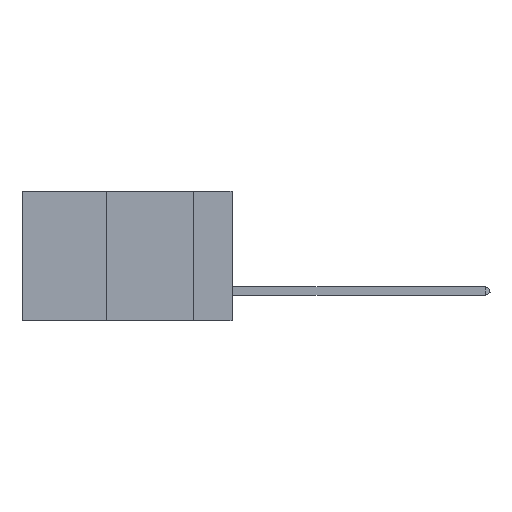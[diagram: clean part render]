
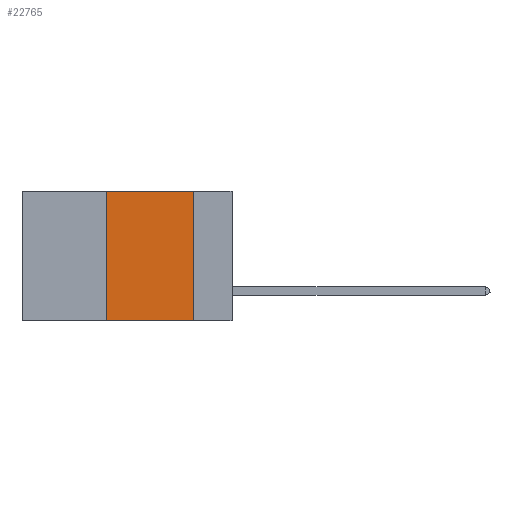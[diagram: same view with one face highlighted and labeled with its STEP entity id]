
A CAD part, left-side view. The second image highlights one B-rep face of the part: STEP entity #22765.
In plain terms, the highlighted planar face has unit normal (-1, 0, 0).
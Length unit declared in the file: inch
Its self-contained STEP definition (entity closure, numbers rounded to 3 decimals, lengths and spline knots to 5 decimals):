
#285 = CARTESIAN_POINT ( 'NONE',  ( 0., 0.36, 0. ) ) ;
#1268 = EDGE_CURVE ( 'NONE', #4175, #27705, #3496, .T. ) ;
#1612 = ORIENTED_EDGE ( 'NONE', *, *, #19260, .T. ) ;
#3496 = LINE ( 'NONE', #9927, #7788 ) ;
#3873 = CARTESIAN_POINT ( 'NONE',  ( 0., 0.6, 0. ) ) ;
#3960 = LINE ( 'NONE', #13238, #23013 ) ;
#4175 = VERTEX_POINT ( 'NONE', #4327 ) ;
#4327 = CARTESIAN_POINT ( 'NONE',  ( 0., 0.36, -0.37 ) ) ;
#4957 = ORIENTED_EDGE ( 'NONE', *, *, #25361, .F. ) ;
#6065 = LINE ( 'NONE', #6774, #22025 ) ;
#6774 = CARTESIAN_POINT ( 'NONE',  ( 0., 0.6, -0.37 ) ) ;
#7014 = CARTESIAN_POINT ( 'NONE',  ( 0., 0.11, 0. ) ) ;
#7085 = LINE ( 'NONE', #27967, #12514 ) ;
#7788 = VECTOR ( 'NONE', #26935, 39.37008 ) ;
#8026 = FACE_OUTER_BOUND ( 'NONE', #24713, .T. ) ;
#8682 = DIRECTION ( 'NONE',  ( 0., 0., -1. ) ) ;
#9927 = CARTESIAN_POINT ( 'NONE',  ( 0., 0.36, 0. ) ) ;
#10274 = AXIS2_PLACEMENT_3D ( 'NONE', #3873, #18843, #8682 ) ;
#10281 = CARTESIAN_POINT ( 'NONE',  ( 0., 0.11, -0.37 ) ) ;
#10612 = DIRECTION ( 'NONE',  ( 0., 0., -1. ) ) ;
#10900 = VERTEX_POINT ( 'NONE', #7014 ) ;
#12514 = VECTOR ( 'NONE', #17991, 39.37008 ) ;
#12987 = PLANE ( 'NONE',  #10274 ) ;
#13238 = CARTESIAN_POINT ( 'NONE',  ( 0., 0.11, 0. ) ) ;
#17991 = DIRECTION ( 'NONE',  ( 0., -1., 0. ) ) ;
#18843 = DIRECTION ( 'NONE',  ( 1., 0., 0. ) ) ;
#19260 = EDGE_CURVE ( 'NONE', #4175, #20201, #6065, .T. ) ;
#20201 = VERTEX_POINT ( 'NONE', #10281 ) ;
#22025 = VECTOR ( 'NONE', #26802, 39.37008 ) ;
#22041 = ORIENTED_EDGE ( 'NONE', *, *, #1268, .F. ) ;
#22765 = ADVANCED_FACE ( 'NONE', ( #8026 ), #12987, .F. ) ;
#23013 = VECTOR ( 'NONE', #10612, 39.37008 ) ;
#24713 = EDGE_LOOP ( 'NONE', ( #4957, #25894, #22041, #1612 ) ) ;
#25075 = EDGE_CURVE ( 'NONE', #27705, #10900, #7085, .T. ) ;
#25361 = EDGE_CURVE ( 'NONE', #10900, #20201, #3960, .T. ) ;
#25894 = ORIENTED_EDGE ( 'NONE', *, *, #25075, .F. ) ;
#26802 = DIRECTION ( 'NONE',  ( 0., -1., 0. ) ) ;
#26935 = DIRECTION ( 'NONE',  ( 0., 0., 1. ) ) ;
#27705 = VERTEX_POINT ( 'NONE', #285 ) ;
#27967 = CARTESIAN_POINT ( 'NONE',  ( 0., 0.6, 0. ) ) ;
